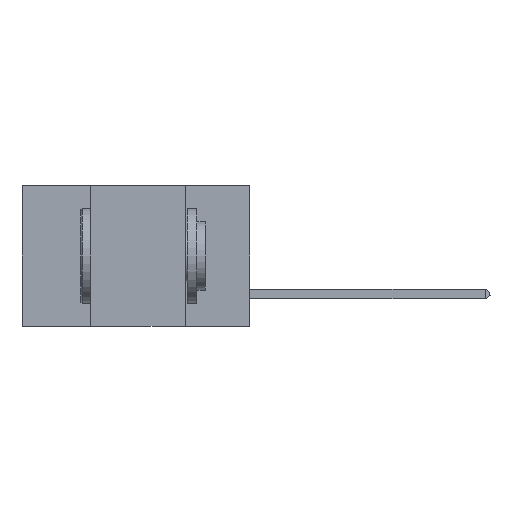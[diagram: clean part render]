
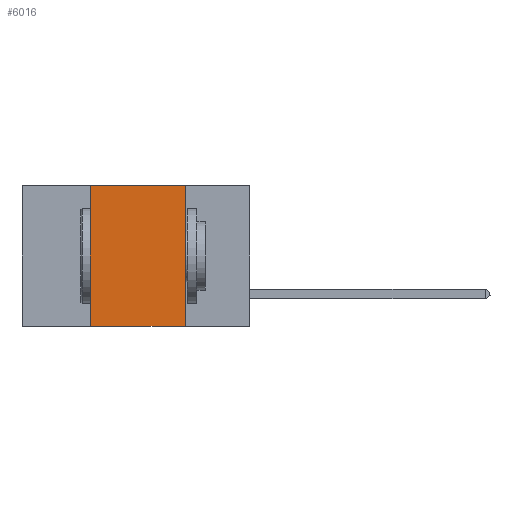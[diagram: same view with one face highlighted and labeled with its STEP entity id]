
A CAD part, left-side view. The second image highlights one B-rep face of the part: STEP entity #6016.
In plain terms, the highlighted planar face has unit normal (-1, 0, 0).
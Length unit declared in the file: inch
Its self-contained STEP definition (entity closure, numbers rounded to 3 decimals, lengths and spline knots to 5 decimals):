
#130 = EDGE_CURVE ( 'NONE', #6630, #4146, #314, .T. ) ;
#216 = ORIENTED_EDGE ( 'NONE', *, *, #3804, .F. ) ;
#314 = LINE ( 'NONE', #9120, #420 ) ;
#360 = DIRECTION ( 'NONE',  ( 0., -1., 0. ) ) ;
#420 = VECTOR ( 'NONE', #360, 39.37008 ) ;
#1498 = VECTOR ( 'NONE', #2093, 39.37008 ) ;
#1680 = ORIENTED_EDGE ( 'NONE', *, *, #4538, .F. ) ;
#1780 = CARTESIAN_POINT ( 'NONE',  ( 0., 0.17, -0.37 ) ) ;
#1852 = LINE ( 'NONE', #5220, #9113 ) ;
#2093 = DIRECTION ( 'NONE',  ( 0., -1., 0. ) ) ;
#2313 = CARTESIAN_POINT ( 'NONE',  ( 0., 0.6, 0. ) ) ;
#2314 = DIRECTION ( 'NONE',  ( 0., 0., -1. ) ) ;
#2416 = DIRECTION ( 'NONE',  ( 0., 0., -1. ) ) ;
#2872 = AXIS2_PLACEMENT_3D ( 'NONE', #2313, #6030, #2416 ) ;
#3709 = EDGE_CURVE ( 'NONE', #5577, #6923, #3932, .T. ) ;
#3804 = EDGE_CURVE ( 'NONE', #4146, #6923, #1852, .T. ) ;
#3932 = LINE ( 'NONE', #8042, #1498 ) ;
#4146 = VERTEX_POINT ( 'NONE', #5319 ) ;
#4244 = CARTESIAN_POINT ( 'NONE',  ( 0., 0.42, -0.37 ) ) ;
#4461 = FACE_OUTER_BOUND ( 'NONE', #8003, .T. ) ;
#4538 = EDGE_CURVE ( 'NONE', #5577, #6630, #4598, .T. ) ;
#4598 = LINE ( 'NONE', #4932, #8073 ) ;
#4932 = CARTESIAN_POINT ( 'NONE',  ( 0., 0.42, 0. ) ) ;
#5220 = CARTESIAN_POINT ( 'NONE',  ( 0., 0.17, 0. ) ) ;
#5319 = CARTESIAN_POINT ( 'NONE',  ( 0., 0.17, 0. ) ) ;
#5577 = VERTEX_POINT ( 'NONE', #4244 ) ;
#5997 = DIRECTION ( 'NONE',  ( 0., 0., 1. ) ) ;
#6016 = ADVANCED_FACE ( 'NONE', ( #4461 ), #6064, .F. ) ;
#6030 = DIRECTION ( 'NONE',  ( 1., 0., 0. ) ) ;
#6064 = PLANE ( 'NONE',  #2872 ) ;
#6630 = VERTEX_POINT ( 'NONE', #7134 ) ;
#6913 = ORIENTED_EDGE ( 'NONE', *, *, #3709, .T. ) ;
#6923 = VERTEX_POINT ( 'NONE', #1780 ) ;
#7134 = CARTESIAN_POINT ( 'NONE',  ( 0., 0.42, 0. ) ) ;
#7237 = ORIENTED_EDGE ( 'NONE', *, *, #130, .F. ) ;
#8003 = EDGE_LOOP ( 'NONE', ( #216, #7237, #1680, #6913 ) ) ;
#8042 = CARTESIAN_POINT ( 'NONE',  ( 0., 0.6, -0.37 ) ) ;
#8073 = VECTOR ( 'NONE', #5997, 39.37008 ) ;
#9113 = VECTOR ( 'NONE', #2314, 39.37008 ) ;
#9120 = CARTESIAN_POINT ( 'NONE',  ( 0., 0.6, 0. ) ) ;
